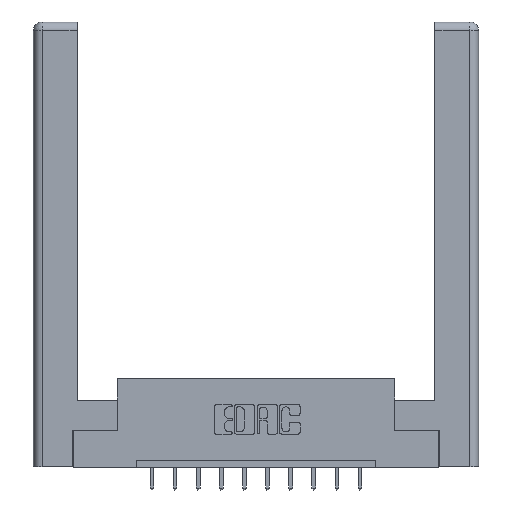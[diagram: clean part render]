
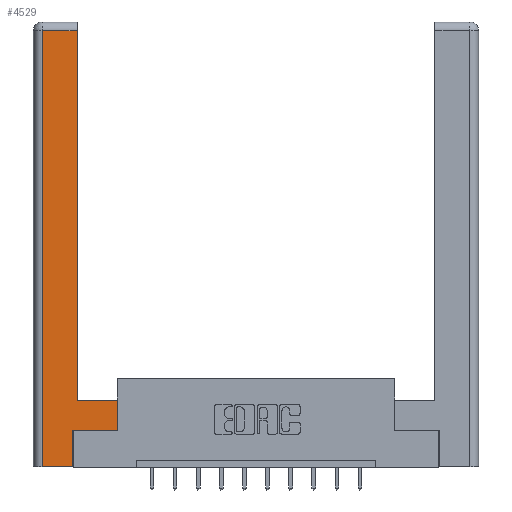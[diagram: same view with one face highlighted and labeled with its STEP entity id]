
A CAD part, top view. The second image highlights one B-rep face of the part: STEP entity #4529.
In plain terms, the highlighted planar face has unit normal (0, 0, 1).
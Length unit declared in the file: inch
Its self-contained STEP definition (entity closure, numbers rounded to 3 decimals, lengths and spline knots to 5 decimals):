
#2 = ORIENTED_EDGE ( 'NONE', *, *, #8585, .T. ) ;
#19 = AXIS2_PLACEMENT_3D ( 'NONE', #12528, #7251, #13697 ) ;
#227 = CARTESIAN_POINT ( 'NONE',  ( 0.265, 0., 0. ) ) ;
#601 = EDGE_CURVE ( 'NONE', #13344, #13849, #3869, .T. ) ;
#631 = LINE ( 'NONE', #10933, #6137 ) ;
#893 = CARTESIAN_POINT ( 'NONE',  ( 0.0615, 0., 0. ) ) ;
#1028 = VERTEX_POINT ( 'NONE', #13013 ) ;
#1163 = ORIENTED_EDGE ( 'NONE', *, *, #10279, .T. ) ;
#1187 = ORIENTED_EDGE ( 'NONE', *, *, #11924, .T. ) ;
#1306 = CARTESIAN_POINT ( 'NONE',  ( 0.0615, 2.94, 0. ) ) ;
#1371 = ORIENTED_EDGE ( 'NONE', *, *, #10451, .T. ) ;
#1521 = CARTESIAN_POINT ( 'NONE',  ( 0.565, 0.45, 0. ) ) ;
#1766 = LINE ( 'NONE', #1306, #6536 ) ;
#2790 = PLANE ( 'NONE',  #19 ) ;
#2797 = DIRECTION ( 'NONE',  ( -1., 0., 0. ) ) ;
#3068 = EDGE_CURVE ( 'NONE', #1028, #5486, #12903, .T. ) ;
#3075 = CARTESIAN_POINT ( 'NONE',  ( 0.0615, 2.94, 0. ) ) ;
#3184 = VERTEX_POINT ( 'NONE', #11711 ) ;
#3411 = VERTEX_POINT ( 'NONE', #3075 ) ;
#3869 = LINE ( 'NONE', #7822, #10891 ) ;
#4038 = ORIENTED_EDGE ( 'NONE', *, *, #601, .T. ) ;
#4188 = VECTOR ( 'NONE', #2797, 39.37008 ) ;
#4529 = ADVANCED_FACE ( 'NONE', ( #11473 ), #2790, .F. ) ;
#4690 = ORIENTED_EDGE ( 'NONE', *, *, #10204, .T. ) ;
#4801 = CARTESIAN_POINT ( 'NONE',  ( 0.565, 0.45, 0. ) ) ;
#4968 = EDGE_CURVE ( 'NONE', #3184, #13344, #5774, .T. ) ;
#5423 = VECTOR ( 'NONE', #11099, 39.37008 ) ;
#5470 = DIRECTION ( 'NONE',  ( 0., 1., 0. ) ) ;
#5486 = VERTEX_POINT ( 'NONE', #4801 ) ;
#5574 = DIRECTION ( 'NONE',  ( 0., 1., 0. ) ) ;
#5774 = LINE ( 'NONE', #9961, #5423 ) ;
#5879 = DIRECTION ( 'NONE',  ( 0., 1., 0. ) ) ;
#6137 = VECTOR ( 'NONE', #5470, 39.37008 ) ;
#6220 = VECTOR ( 'NONE', #9895, 39.37008 ) ;
#6536 = VECTOR ( 'NONE', #8928, 39.37008 ) ;
#7251 = DIRECTION ( 'NONE',  ( 0., 0., -1. ) ) ;
#7351 = CARTESIAN_POINT ( 'NONE',  ( 0.295, 0.45, 0. ) ) ;
#7507 = CARTESIAN_POINT ( 'NONE',  ( 0.565, 0.245, 0. ) ) ;
#7822 = CARTESIAN_POINT ( 'NONE',  ( 0.265, 0.245, 0. ) ) ;
#8067 = VERTEX_POINT ( 'NONE', #14092 ) ;
#8354 = ORIENTED_EDGE ( 'NONE', *, *, #4968, .T. ) ;
#8585 = EDGE_CURVE ( 'NONE', #5486, #8067, #9374, .T. ) ;
#8683 = DIRECTION ( 'NONE',  ( 1., 0., 0. ) ) ;
#8928 = DIRECTION ( 'NONE',  ( -1., 0., 0. ) ) ;
#9374 = LINE ( 'NONE', #7351, #4188 ) ;
#9895 = DIRECTION ( 'NONE',  ( 0., -1., 0. ) ) ;
#9961 = CARTESIAN_POINT ( 'NONE',  ( 0.265, 0., 0. ) ) ;
#10204 = EDGE_CURVE ( 'NONE', #3411, #3184, #13081, .T. ) ;
#10279 = EDGE_CURVE ( 'NONE', #13849, #1028, #12755, .T. ) ;
#10451 = EDGE_CURVE ( 'NONE', #13292, #3411, #1766, .T. ) ;
#10539 = VECTOR ( 'NONE', #8683, 39.37008 ) ;
#10891 = VECTOR ( 'NONE', #5574, 39.37008 ) ;
#10933 = CARTESIAN_POINT ( 'NONE',  ( 0.295, 3., 0. ) ) ;
#10948 = CARTESIAN_POINT ( 'NONE',  ( 0.265, 0.245, 0. ) ) ;
#11099 = DIRECTION ( 'NONE',  ( 1., 0., 0. ) ) ;
#11473 = FACE_OUTER_BOUND ( 'NONE', #13208, .T. ) ;
#11711 = CARTESIAN_POINT ( 'NONE',  ( 0.0615, 0., 0. ) ) ;
#11924 = EDGE_CURVE ( 'NONE', #8067, #13292, #631, .T. ) ;
#12174 = CARTESIAN_POINT ( 'NONE',  ( 0.295, 2.94, 0. ) ) ;
#12528 = CARTESIAN_POINT ( 'NONE',  ( 0., 0., 0. ) ) ;
#12549 = VECTOR ( 'NONE', #5879, 39.37008 ) ;
#12755 = LINE ( 'NONE', #7507, #10539 ) ;
#12903 = LINE ( 'NONE', #1521, #12549 ) ;
#13013 = CARTESIAN_POINT ( 'NONE',  ( 0.565, 0.245, 0. ) ) ;
#13081 = LINE ( 'NONE', #893, #6220 ) ;
#13208 = EDGE_LOOP ( 'NONE', ( #1187, #1371, #4690, #8354, #4038, #1163, #13843, #2 ) ) ;
#13292 = VERTEX_POINT ( 'NONE', #12174 ) ;
#13344 = VERTEX_POINT ( 'NONE', #227 ) ;
#13697 = DIRECTION ( 'NONE',  ( -1., 0., 0. ) ) ;
#13843 = ORIENTED_EDGE ( 'NONE', *, *, #3068, .T. ) ;
#13849 = VERTEX_POINT ( 'NONE', #10948 ) ;
#14092 = CARTESIAN_POINT ( 'NONE',  ( 0.295, 0.45, 0. ) ) ;
